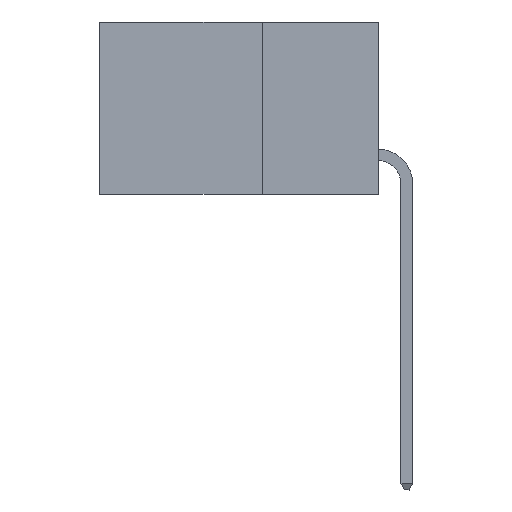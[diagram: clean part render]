
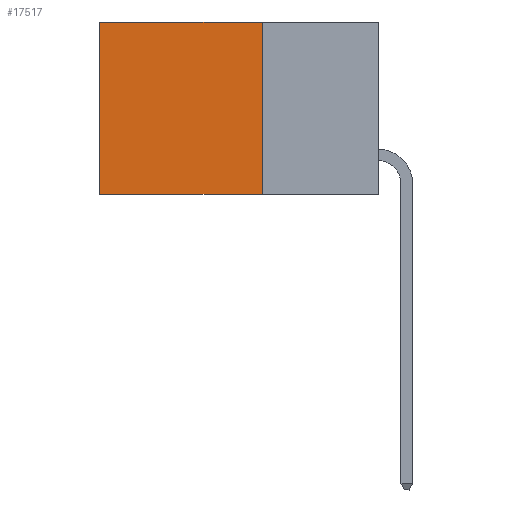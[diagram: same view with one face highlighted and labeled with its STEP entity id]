
A CAD part, left-side view. The second image highlights one B-rep face of the part: STEP entity #17517.
In plain terms, the highlighted planar face has unit normal (-1, 0, 0).
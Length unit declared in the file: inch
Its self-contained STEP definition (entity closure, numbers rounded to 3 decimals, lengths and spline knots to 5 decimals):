
#827 = CARTESIAN_POINT ( 'NONE',  ( 0.2615, 0.6, 0. ) ) ;
#1009 = VECTOR ( 'NONE', #7852, 39.37008 ) ;
#2996 = ORIENTED_EDGE ( 'NONE', *, *, #17265, .T. ) ;
#3246 = FACE_OUTER_BOUND ( 'NONE', #13793, .T. ) ;
#5091 = CARTESIAN_POINT ( 'NONE',  ( 0.2615, 0.25, 0. ) ) ;
#5154 = CARTESIAN_POINT ( 'NONE',  ( 0.2615, 0.25, -0.37 ) ) ;
#6271 = VECTOR ( 'NONE', #12163, 39.37008 ) ;
#6734 = EDGE_CURVE ( 'NONE', #19798, #15282, #24187, .T. ) ;
#7698 = PLANE ( 'NONE',  #14267 ) ;
#7852 = DIRECTION ( 'NONE',  ( 0., 0., -1. ) ) ;
#8627 = CARTESIAN_POINT ( 'NONE',  ( 0.2615, 0.25, 0. ) ) ;
#9873 = EDGE_CURVE ( 'NONE', #20550, #19798, #13232, .T. ) ;
#10651 = LINE ( 'NONE', #8627, #17745 ) ;
#10690 = VERTEX_POINT ( 'NONE', #827 ) ;
#11948 = CARTESIAN_POINT ( 'NONE',  ( 0.2615, 0.6, -0.37 ) ) ;
#12163 = DIRECTION ( 'NONE',  ( 0., 1., 0. ) ) ;
#13232 = LINE ( 'NONE', #21191, #16104 ) ;
#13364 = CARTESIAN_POINT ( 'NONE',  ( 0.2615, 0.6, -0.37 ) ) ;
#13793 = EDGE_LOOP ( 'NONE', ( #2996, #20518, #16976, #16237 ) ) ;
#14260 = CARTESIAN_POINT ( 'NONE',  ( 0.2615, 0.25, -0.37 ) ) ;
#14267 = AXIS2_PLACEMENT_3D ( 'NONE', #23075, #18990, #21584 ) ;
#15282 = VERTEX_POINT ( 'NONE', #13364 ) ;
#16104 = VECTOR ( 'NONE', #24366, 39.37008 ) ;
#16237 = ORIENTED_EDGE ( 'NONE', *, *, #20490, .T. ) ;
#16976 = ORIENTED_EDGE ( 'NONE', *, *, #9873, .F. ) ;
#17265 = EDGE_CURVE ( 'NONE', #10690, #15282, #20307, .T. ) ;
#17517 = ADVANCED_FACE ( 'NONE', ( #3246 ), #7698, .F. ) ;
#17745 = VECTOR ( 'NONE', #24634, 39.37008 ) ;
#18990 = DIRECTION ( 'NONE',  ( 1., 0., 0. ) ) ;
#19798 = VERTEX_POINT ( 'NONE', #5154 ) ;
#20307 = LINE ( 'NONE', #11948, #1009 ) ;
#20490 = EDGE_CURVE ( 'NONE', #20550, #10690, #10651, .T. ) ;
#20518 = ORIENTED_EDGE ( 'NONE', *, *, #6734, .F. ) ;
#20550 = VERTEX_POINT ( 'NONE', #5091 ) ;
#21191 = CARTESIAN_POINT ( 'NONE',  ( 0.2615, 0.25, -0.37 ) ) ;
#21584 = DIRECTION ( 'NONE',  ( 0., 0., -1. ) ) ;
#23075 = CARTESIAN_POINT ( 'NONE',  ( 0.2615, 0.25, -0.37 ) ) ;
#24187 = LINE ( 'NONE', #14260, #6271 ) ;
#24366 = DIRECTION ( 'NONE',  ( 0., 0., -1. ) ) ;
#24634 = DIRECTION ( 'NONE',  ( 0., 1., 0. ) ) ;
